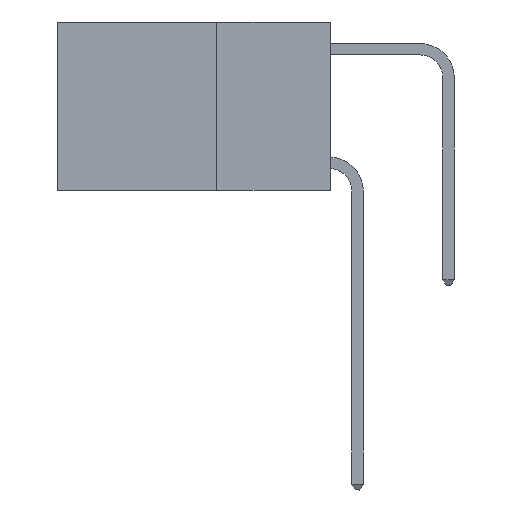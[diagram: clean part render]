
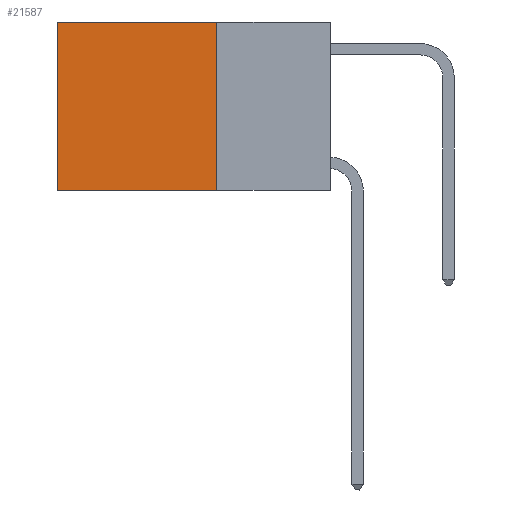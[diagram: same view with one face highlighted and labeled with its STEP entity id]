
A CAD part, left-side view. The second image highlights one B-rep face of the part: STEP entity #21587.
In plain terms, the highlighted planar face has unit normal (-1, 0, 0).
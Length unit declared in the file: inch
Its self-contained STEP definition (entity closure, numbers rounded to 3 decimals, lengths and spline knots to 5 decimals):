
#80 = LINE ( 'NONE', #17523, #6950 ) ;
#575 = EDGE_CURVE ( 'NONE', #9854, #968, #13819, .T. ) ;
#968 = VERTEX_POINT ( 'NONE', #7034 ) ;
#3628 = EDGE_CURVE ( 'NONE', #5891, #9854, #6678, .T. ) ;
#4134 = CARTESIAN_POINT ( 'NONE',  ( 0.2625, 0.25, 0. ) ) ;
#4190 = DIRECTION ( 'NONE',  ( 0., 1., 0. ) ) ;
#4630 = EDGE_CURVE ( 'NONE', #5891, #22937, #5775, .T. ) ;
#5770 = CARTESIAN_POINT ( 'NONE',  ( 0.2625, 0.6, 0. ) ) ;
#5775 = LINE ( 'NONE', #4134, #6391 ) ;
#5891 = VERTEX_POINT ( 'NONE', #21443 ) ;
#6354 = ORIENTED_EDGE ( 'NONE', *, *, #3628, .F. ) ;
#6391 = VECTOR ( 'NONE', #15655, 39.37008 ) ;
#6678 = LINE ( 'NONE', #22113, #19232 ) ;
#6950 = VECTOR ( 'NONE', #7835, 39.37008 ) ;
#7034 = CARTESIAN_POINT ( 'NONE',  ( 0.2625, 0.6, -0.37 ) ) ;
#7835 = DIRECTION ( 'NONE',  ( 0., 0., -1. ) ) ;
#7903 = DIRECTION ( 'NONE',  ( 0., 0., -1. ) ) ;
#9292 = VECTOR ( 'NONE', #4190, 39.37008 ) ;
#9854 = VERTEX_POINT ( 'NONE', #11808 ) ;
#10289 = EDGE_LOOP ( 'NONE', ( #19278, #17989, #6354, #11879 ) ) ;
#11808 = CARTESIAN_POINT ( 'NONE',  ( 0.2625, 0.25, -0.37 ) ) ;
#11879 = ORIENTED_EDGE ( 'NONE', *, *, #4630, .T. ) ;
#11987 = EDGE_CURVE ( 'NONE', #22937, #968, #80, .T. ) ;
#12620 = AXIS2_PLACEMENT_3D ( 'NONE', #22986, #20962, #19285 ) ;
#13037 = FACE_OUTER_BOUND ( 'NONE', #10289, .T. ) ;
#13819 = LINE ( 'NONE', #17808, #9292 ) ;
#15655 = DIRECTION ( 'NONE',  ( 0., 1., 0. ) ) ;
#17523 = CARTESIAN_POINT ( 'NONE',  ( 0.2625, 0.6, 0. ) ) ;
#17808 = CARTESIAN_POINT ( 'NONE',  ( 0.2625, 0.25, -0.37 ) ) ;
#17989 = ORIENTED_EDGE ( 'NONE', *, *, #575, .F. ) ;
#19232 = VECTOR ( 'NONE', #7903, 39.37008 ) ;
#19278 = ORIENTED_EDGE ( 'NONE', *, *, #11987, .T. ) ;
#19285 = DIRECTION ( 'NONE',  ( 0., 0., -1. ) ) ;
#20962 = DIRECTION ( 'NONE',  ( 1., 0., 0. ) ) ;
#21201 = PLANE ( 'NONE',  #12620 ) ;
#21443 = CARTESIAN_POINT ( 'NONE',  ( 0.2625, 0.25, 0. ) ) ;
#21587 = ADVANCED_FACE ( 'NONE', ( #13037 ), #21201, .F. ) ;
#22113 = CARTESIAN_POINT ( 'NONE',  ( 0.2625, 0.25, 0. ) ) ;
#22937 = VERTEX_POINT ( 'NONE', #5770 ) ;
#22986 = CARTESIAN_POINT ( 'NONE',  ( 0.2625, 0.25, 0. ) ) ;
